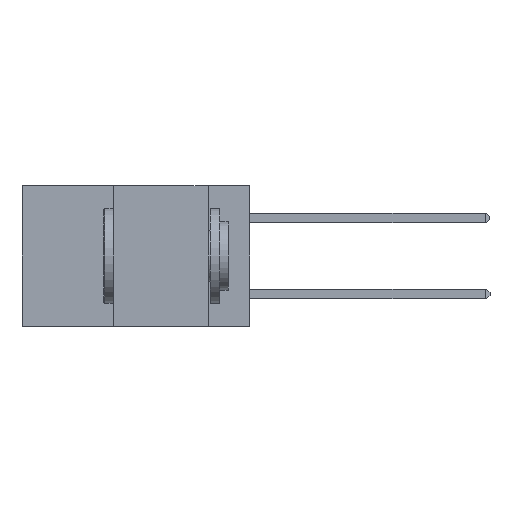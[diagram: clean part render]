
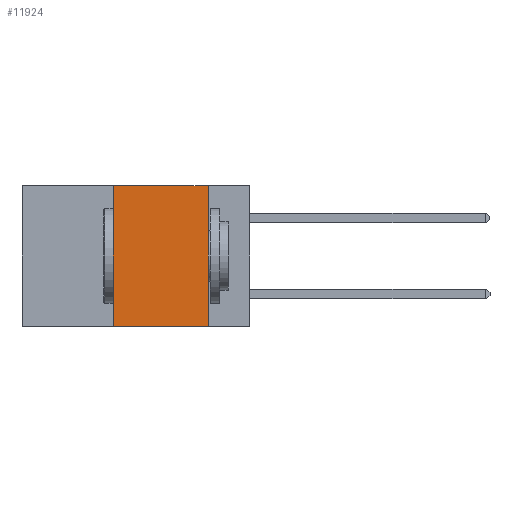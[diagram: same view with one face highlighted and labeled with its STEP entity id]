
A CAD part, left-side view. The second image highlights one B-rep face of the part: STEP entity #11924.
In plain terms, the highlighted planar face has unit normal (-1, 0, 0).
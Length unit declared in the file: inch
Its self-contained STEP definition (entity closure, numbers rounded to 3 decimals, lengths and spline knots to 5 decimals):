
#204 = EDGE_CURVE ( 'NONE', #6793, #2746, #17289, .T. ) ;
#473 = DIRECTION ( 'NONE',  ( 0., -1., 0. ) ) ;
#511 = AXIS2_PLACEMENT_3D ( 'NONE', #14824, #4008, #16597 ) ;
#1153 = CARTESIAN_POINT ( 'NONE',  ( 0., 0.36, -0.37 ) ) ;
#1478 = CARTESIAN_POINT ( 'NONE',  ( 0., 0.11, 0. ) ) ;
#1819 = VECTOR ( 'NONE', #20677, 39.37008 ) ;
#2033 = LINE ( 'NONE', #4641, #16398 ) ;
#2746 = VERTEX_POINT ( 'NONE', #6409 ) ;
#2950 = VECTOR ( 'NONE', #8444, 39.37008 ) ;
#4008 = DIRECTION ( 'NONE',  ( 1., 0., 0. ) ) ;
#4641 = CARTESIAN_POINT ( 'NONE',  ( 0., 0.11, 0. ) ) ;
#6409 = CARTESIAN_POINT ( 'NONE',  ( 0., 0.11, -0.37 ) ) ;
#6793 = VERTEX_POINT ( 'NONE', #1153 ) ;
#7090 = LINE ( 'NONE', #21990, #11297 ) ;
#7146 = ORIENTED_EDGE ( 'NONE', *, *, #18060, .F. ) ;
#7973 = CARTESIAN_POINT ( 'NONE',  ( 0., 0.6, -0.37 ) ) ;
#8084 = CARTESIAN_POINT ( 'NONE',  ( 0., 0.36, 0. ) ) ;
#8428 = EDGE_LOOP ( 'NONE', ( #18683, #10545, #7146, #20643 ) ) ;
#8444 = DIRECTION ( 'NONE',  ( 0., -1., 0. ) ) ;
#10545 = ORIENTED_EDGE ( 'NONE', *, *, #19781, .F. ) ;
#11297 = VECTOR ( 'NONE', #473, 39.37008 ) ;
#11924 = ADVANCED_FACE ( 'NONE', ( #21462 ), #14749, .F. ) ;
#11964 = LINE ( 'NONE', #8084, #1819 ) ;
#12174 = EDGE_CURVE ( 'NONE', #18278, #2746, #2033, .T. ) ;
#13887 = VERTEX_POINT ( 'NONE', #21706 ) ;
#14749 = PLANE ( 'NONE',  #511 ) ;
#14824 = CARTESIAN_POINT ( 'NONE',  ( 0., 0.6, 0. ) ) ;
#15464 = DIRECTION ( 'NONE',  ( 0., 0., -1. ) ) ;
#16398 = VECTOR ( 'NONE', #15464, 39.37008 ) ;
#16597 = DIRECTION ( 'NONE',  ( 0., 0., -1. ) ) ;
#17289 = LINE ( 'NONE', #7973, #2950 ) ;
#18060 = EDGE_CURVE ( 'NONE', #6793, #13887, #11964, .T. ) ;
#18278 = VERTEX_POINT ( 'NONE', #1478 ) ;
#18683 = ORIENTED_EDGE ( 'NONE', *, *, #12174, .F. ) ;
#19781 = EDGE_CURVE ( 'NONE', #13887, #18278, #7090, .T. ) ;
#20643 = ORIENTED_EDGE ( 'NONE', *, *, #204, .T. ) ;
#20677 = DIRECTION ( 'NONE',  ( 0., 0., 1. ) ) ;
#21462 = FACE_OUTER_BOUND ( 'NONE', #8428, .T. ) ;
#21706 = CARTESIAN_POINT ( 'NONE',  ( 0., 0.36, 0. ) ) ;
#21990 = CARTESIAN_POINT ( 'NONE',  ( 0., 0.6, 0. ) ) ;
